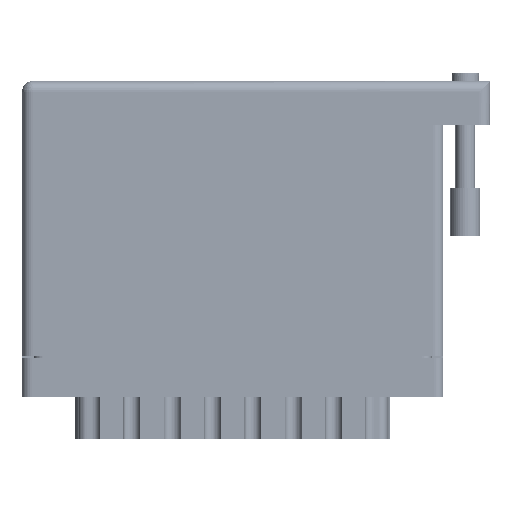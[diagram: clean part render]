
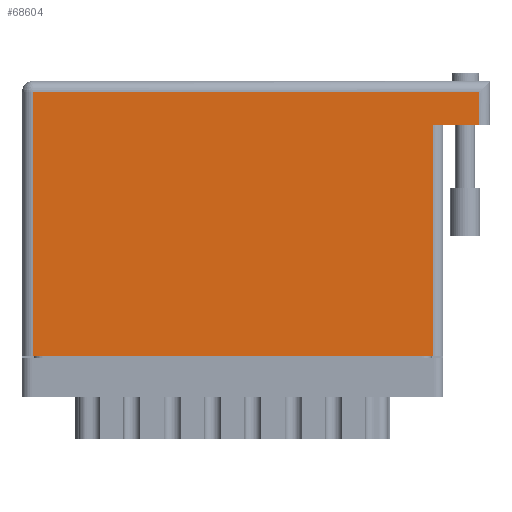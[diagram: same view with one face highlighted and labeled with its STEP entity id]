
A CAD part, front view. The second image highlights one B-rep face of the part: STEP entity #68604.
In plain terms, the highlighted face is planar.
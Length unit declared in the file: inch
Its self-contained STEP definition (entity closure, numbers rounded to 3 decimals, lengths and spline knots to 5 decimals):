
#158 = CARTESIAN_POINT ( 'NONE',  ( 2.648, 1.495, 0. ) ) ;
#636 = EDGE_CURVE ( 'NONE', #37827, #28775, #5877, .T. ) ;
#2299 = AXIS2_PLACEMENT_3D ( 'NONE', #27065, #4231, #55220 ) ;
#2762 = VERTEX_POINT ( 'NONE', #45474 ) ;
#4231 = DIRECTION ( 'NONE',  ( 0., 0., -1. ) ) ;
#4342 = EDGE_CURVE ( 'NONE', #24332, #38649, #17797, .T. ) ;
#4420 = FACE_OUTER_BOUND ( 'NONE', #32914, .T. ) ;
#5474 = VECTOR ( 'NONE', #16307, 39.37008 ) ;
#5777 = CARTESIAN_POINT ( 'NONE',  ( 2.948, 1.775, 0. ) ) ;
#5877 = LINE ( 'NONE', #52721, #62985 ) ;
#8757 = CARTESIAN_POINT ( 'NONE',  ( 0., 0., 0. ) ) ;
#9678 = ORIENTED_EDGE ( 'NONE', *, *, #51333, .T. ) ;
#10058 = DIRECTION ( 'NONE',  ( -1., 0., 0. ) ) ;
#11933 = LINE ( 'NONE', #24807, #32104 ) ;
#14756 = DIRECTION ( 'NONE',  ( 0., -1., 0. ) ) ;
#16237 = CARTESIAN_POINT ( 'NONE',  ( 3.018, 1.495, 0. ) ) ;
#16307 = DIRECTION ( 'NONE',  ( 0., 1., 0. ) ) ;
#17797 = LINE ( 'NONE', #16237, #62522 ) ;
#18487 = ORIENTED_EDGE ( 'NONE', *, *, #4342, .F. ) ;
#20324 = DIRECTION ( 'NONE',  ( 1., 0., 0. ) ) ;
#23652 = CARTESIAN_POINT ( 'NONE',  ( 2.948, 1.495, 0. ) ) ;
#24332 = VERTEX_POINT ( 'NONE', #23652 ) ;
#24461 = ORIENTED_EDGE ( 'NONE', *, *, #38581, .T. ) ;
#24807 = CARTESIAN_POINT ( 'NONE',  ( 0.07, 0., 0. ) ) ;
#25465 = ORIENTED_EDGE ( 'NONE', *, *, #636, .T. ) ;
#27065 = CARTESIAN_POINT ( 'NONE',  ( 0., 1.775, 0. ) ) ;
#28775 = VERTEX_POINT ( 'NONE', #46329 ) ;
#31818 = LINE ( 'NONE', #60902, #5474 ) ;
#32104 = VECTOR ( 'NONE', #14756, 39.37008 ) ;
#32914 = EDGE_LOOP ( 'NONE', ( #51645, #9678, #18487, #24461, #25465, #71984 ) ) ;
#32999 = EDGE_CURVE ( 'NONE', #28775, #2762, #11933, .T. ) ;
#34225 = DIRECTION ( 'NONE',  ( 0., 1., 0. ) ) ;
#37800 = PLANE ( 'NONE',  #2299 ) ;
#37827 = VERTEX_POINT ( 'NONE', #61084 ) ;
#38581 = EDGE_CURVE ( 'NONE', #24332, #37827, #62770, .T. ) ;
#38649 = VERTEX_POINT ( 'NONE', #158 ) ;
#39521 = LINE ( 'NONE', #8757, #54453 ) ;
#41969 = VERTEX_POINT ( 'NONE', #65845 ) ;
#42516 = VECTOR ( 'NONE', #34225, 39.37008 ) ;
#45474 = CARTESIAN_POINT ( 'NONE',  ( 0.07, 0., 0. ) ) ;
#46329 = CARTESIAN_POINT ( 'NONE',  ( 0.07, 1.705, 0. ) ) ;
#51333 = EDGE_CURVE ( 'NONE', #41969, #38649, #31818, .T. ) ;
#51645 = ORIENTED_EDGE ( 'NONE', *, *, #52584, .T. ) ;
#52584 = EDGE_CURVE ( 'NONE', #2762, #41969, #39521, .T. ) ;
#52721 = CARTESIAN_POINT ( 'NONE',  ( 0., 1.705, 0. ) ) ;
#54453 = VECTOR ( 'NONE', #20324, 39.37008 ) ;
#55220 = DIRECTION ( 'NONE',  ( -1., 0., 0. ) ) ;
#60902 = CARTESIAN_POINT ( 'NONE',  ( 2.648, 1.495, 0. ) ) ;
#61084 = CARTESIAN_POINT ( 'NONE',  ( 2.948, 1.705, 0. ) ) ;
#62522 = VECTOR ( 'NONE', #10058, 39.37008 ) ;
#62770 = LINE ( 'NONE', #5777, #42516 ) ;
#62985 = VECTOR ( 'NONE', #70931, 39.37008 ) ;
#65845 = CARTESIAN_POINT ( 'NONE',  ( 2.648, 0., 0. ) ) ;
#68604 = ADVANCED_FACE ( 'NONE', ( #4420 ), #37800, .F. ) ;
#70931 = DIRECTION ( 'NONE',  ( -1., 0., 0. ) ) ;
#71984 = ORIENTED_EDGE ( 'NONE', *, *, #32999, .T. ) ;
